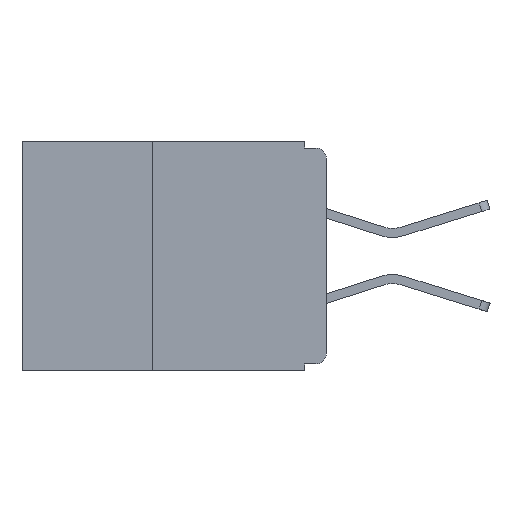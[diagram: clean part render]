
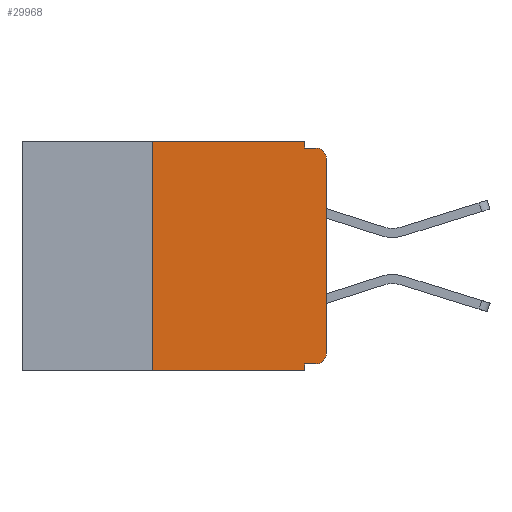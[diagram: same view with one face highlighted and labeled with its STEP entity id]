
A CAD part, left-side view. The second image highlights one B-rep face of the part: STEP entity #29968.
In plain terms, the highlighted planar face has unit normal (-1, 0, 0).
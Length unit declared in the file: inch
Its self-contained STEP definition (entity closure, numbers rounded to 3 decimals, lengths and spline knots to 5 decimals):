
#30 = DIRECTION ( 'NONE',  ( 0., -1., 0. ) ) ;
#329 = VERTEX_POINT ( 'NONE', #17840 ) ;
#393 = CARTESIAN_POINT ( 'NONE',  ( 0., 0.031, -0.32 ) ) ;
#778 = DIRECTION ( 'NONE',  ( 0., -1., 0. ) ) ;
#1935 = DIRECTION ( 'NONE',  ( 1., 0., 0. ) ) ;
#3013 = EDGE_CURVE ( 'NONE', #21777, #5148, #24240, .T. ) ;
#3023 = VECTOR ( 'NONE', #778, 39.37008 ) ;
#3149 = DIRECTION ( 'NONE',  ( 0., 0., -1. ) ) ;
#3760 = EDGE_CURVE ( 'NONE', #22274, #5148, #34524, .T. ) ;
#3877 = CARTESIAN_POINT ( 'NONE',  ( 0., 0.031, 0. ) ) ;
#3903 = LINE ( 'NONE', #11674, #3023 ) ;
#3972 = CARTESIAN_POINT ( 'NONE',  ( 0., 0., -0.32 ) ) ;
#4036 = DIRECTION ( 'NONE',  ( 0., 0., 1. ) ) ;
#4309 = ORIENTED_EDGE ( 'NONE', *, *, #3013, .T. ) ;
#4663 = CARTESIAN_POINT ( 'NONE',  ( 0., 0.25, 0. ) ) ;
#4811 = EDGE_CURVE ( 'NONE', #21777, #30571, #30337, .T. ) ;
#5148 = VERTEX_POINT ( 'NONE', #33631 ) ;
#6034 = EDGE_CURVE ( 'NONE', #29356, #329, #20257, .T. ) ;
#7422 = EDGE_CURVE ( 'NONE', #14850, #23898, #31823, .T. ) ;
#8879 = VECTOR ( 'NONE', #26029, 39.37008 ) ;
#8979 = EDGE_CURVE ( 'NONE', #23898, #13992, #16470, .T. ) ;
#9210 = CARTESIAN_POINT ( 'NONE',  ( 0., 0.25, -0.33 ) ) ;
#10336 = CARTESIAN_POINT ( 'NONE',  ( 0., 0.031, 0. ) ) ;
#10618 = CARTESIAN_POINT ( 'NONE',  ( 0., 0.015, -0.025 ) ) ;
#11526 = AXIS2_PLACEMENT_3D ( 'NONE', #10618, #29464, #13375 ) ;
#11674 = CARTESIAN_POINT ( 'NONE',  ( 0., 0.437, 0. ) ) ;
#12795 = PLANE ( 'NONE',  #26401 ) ;
#13375 = DIRECTION ( 'NONE',  ( 0., 0., -1. ) ) ;
#13992 = VERTEX_POINT ( 'NONE', #20887 ) ;
#14749 = CARTESIAN_POINT ( 'NONE',  ( 0., 0.015, -0.01 ) ) ;
#14850 = VERTEX_POINT ( 'NONE', #34705 ) ;
#15197 = VECTOR ( 'NONE', #28318, 39.37008 ) ;
#15354 = AXIS2_PLACEMENT_3D ( 'NONE', #24252, #24148, #24020 ) ;
#15549 = CARTESIAN_POINT ( 'NONE',  ( 0., 0.437, 0. ) ) ;
#15887 = EDGE_CURVE ( 'NONE', #14850, #22274, #22400, .T. ) ;
#16236 = VECTOR ( 'NONE', #30, 39.37008 ) ;
#16470 = LINE ( 'NONE', #23039, #30708 ) ;
#17840 = CARTESIAN_POINT ( 'NONE',  ( 0., 0.031, -0.01 ) ) ;
#18055 = EDGE_CURVE ( 'NONE', #30571, #29356, #3903, .T. ) ;
#18255 = CIRCLE ( 'NONE', #11526, 0.015 ) ;
#18321 = ORIENTED_EDGE ( 'NONE', *, *, #4811, .F. ) ;
#18733 = ORIENTED_EDGE ( 'NONE', *, *, #6034, .F. ) ;
#19395 = VECTOR ( 'NONE', #3149, 39.37008 ) ;
#19621 = EDGE_CURVE ( 'NONE', #329, #31594, #21848, .T. ) ;
#20257 = LINE ( 'NONE', #3877, #19395 ) ;
#20280 = DIRECTION ( 'NONE',  ( 0., 0., -1. ) ) ;
#20385 = CARTESIAN_POINT ( 'NONE',  ( 0., 0.031, -0.33 ) ) ;
#20442 = ORIENTED_EDGE ( 'NONE', *, *, #18055, .F. ) ;
#20478 = ORIENTED_EDGE ( 'NONE', *, *, #3760, .F. ) ;
#20887 = CARTESIAN_POINT ( 'NONE',  ( 0., 0., -0.025 ) ) ;
#20999 = VECTOR ( 'NONE', #23650, 39.37008 ) ;
#21000 = DIRECTION ( 'NONE',  ( 0., 0., -1. ) ) ;
#21777 = VERTEX_POINT ( 'NONE', #9210 ) ;
#21848 = LINE ( 'NONE', #28986, #20999 ) ;
#22274 = VERTEX_POINT ( 'NONE', #393 ) ;
#22400 = LINE ( 'NONE', #3972, #15197 ) ;
#23039 = CARTESIAN_POINT ( 'NONE',  ( 0., 0., 0. ) ) ;
#23106 = CARTESIAN_POINT ( 'NONE',  ( 0., 0.437, -0.33 ) ) ;
#23412 = FACE_OUTER_BOUND ( 'NONE', #24395, .T. ) ;
#23650 = DIRECTION ( 'NONE',  ( 0., -1., 0. ) ) ;
#23898 = VERTEX_POINT ( 'NONE', #26387 ) ;
#24020 = DIRECTION ( 'NONE',  ( 0., 0., -1. ) ) ;
#24148 = DIRECTION ( 'NONE',  ( -1., 0., 0. ) ) ;
#24240 = LINE ( 'NONE', #23106, #16236 ) ;
#24252 = CARTESIAN_POINT ( 'NONE',  ( 0., 0.015, -0.305 ) ) ;
#24395 = EDGE_LOOP ( 'NONE', ( #26205, #33269, #25813, #18733, #20442, #18321, #4309, #20478, #26742, #33797 ) ) ;
#25813 = ORIENTED_EDGE ( 'NONE', *, *, #19621, .F. ) ;
#26029 = DIRECTION ( 'NONE',  ( 0., 0., 1. ) ) ;
#26205 = ORIENTED_EDGE ( 'NONE', *, *, #8979, .T. ) ;
#26387 = CARTESIAN_POINT ( 'NONE',  ( 0., 0., -0.305 ) ) ;
#26401 = AXIS2_PLACEMENT_3D ( 'NONE', #15549, #1935, #21000 ) ;
#26742 = ORIENTED_EDGE ( 'NONE', *, *, #15887, .F. ) ;
#27504 = VECTOR ( 'NONE', #20280, 39.37008 ) ;
#28318 = DIRECTION ( 'NONE',  ( 0., 1., 0. ) ) ;
#28986 = CARTESIAN_POINT ( 'NONE',  ( 0., 0., -0.01 ) ) ;
#29356 = VERTEX_POINT ( 'NONE', #10336 ) ;
#29464 = DIRECTION ( 'NONE',  ( -1., 0., 0. ) ) ;
#29968 = ADVANCED_FACE ( 'NONE', ( #23412 ), #12795, .F. ) ;
#30337 = LINE ( 'NONE', #30942, #8879 ) ;
#30571 = VERTEX_POINT ( 'NONE', #4663 ) ;
#30708 = VECTOR ( 'NONE', #4036, 39.37008 ) ;
#30942 = CARTESIAN_POINT ( 'NONE',  ( 0., 0.25, -0.33 ) ) ;
#31594 = VERTEX_POINT ( 'NONE', #14749 ) ;
#31673 = EDGE_CURVE ( 'NONE', #13992, #31594, #18255, .T. ) ;
#31823 = CIRCLE ( 'NONE', #15354, 0.015 ) ;
#33269 = ORIENTED_EDGE ( 'NONE', *, *, #31673, .T. ) ;
#33631 = CARTESIAN_POINT ( 'NONE',  ( 0., 0.031, -0.33 ) ) ;
#33797 = ORIENTED_EDGE ( 'NONE', *, *, #7422, .T. ) ;
#34524 = LINE ( 'NONE', #20385, #27504 ) ;
#34705 = CARTESIAN_POINT ( 'NONE',  ( 0., 0.015, -0.32 ) ) ;
